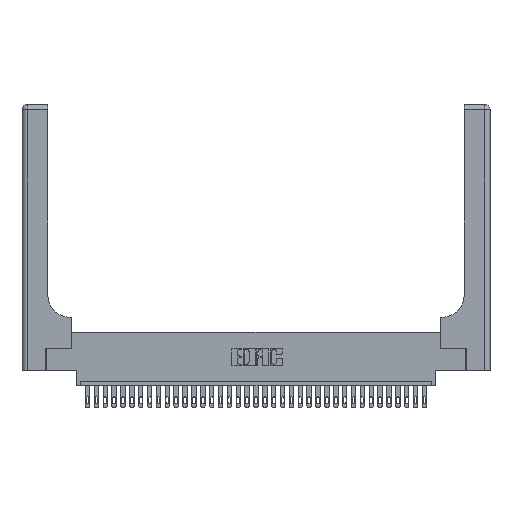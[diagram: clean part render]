
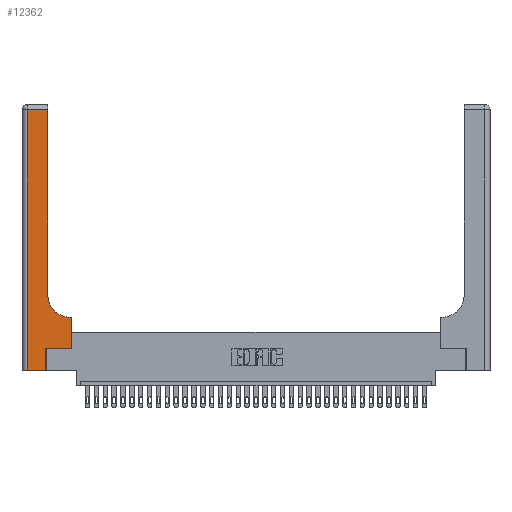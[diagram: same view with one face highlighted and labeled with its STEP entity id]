
A CAD part, top view. The second image highlights one B-rep face of the part: STEP entity #12362.
In plain terms, the highlighted planar face has unit normal (0, 0, 1).
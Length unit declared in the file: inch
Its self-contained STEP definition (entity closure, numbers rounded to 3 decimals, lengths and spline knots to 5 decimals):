
#39 = VECTOR ( 'NONE', #33072, 39.37008 ) ;
#1575 = CARTESIAN_POINT ( 'NONE',  ( 0.06, 0., 0.37 ) ) ;
#1857 = VECTOR ( 'NONE', #12751, 39.37008 ) ;
#2114 = ORIENTED_EDGE ( 'NONE', *, *, #26939, .T. ) ;
#2573 = VERTEX_POINT ( 'NONE', #28068 ) ;
#3101 = CARTESIAN_POINT ( 'NONE',  ( 0.269, 0., 0.37 ) ) ;
#4083 = VECTOR ( 'NONE', #10354, 39.37008 ) ;
#4309 = CARTESIAN_POINT ( 'NONE',  ( 0.2915, 3., 0.37 ) ) ;
#4484 = CARTESIAN_POINT ( 'NONE',  ( 0.2915, 0.85, 0.37 ) ) ;
#4776 = DIRECTION ( 'NONE',  ( 0., -1., 0. ) ) ;
#4898 = CARTESIAN_POINT ( 'NONE',  ( 0.5585, 0.25, 0.37 ) ) ;
#6067 = PLANE ( 'NONE',  #28166 ) ;
#6291 = CARTESIAN_POINT ( 'NONE',  ( 0.5415, 0.85, 0.37 ) ) ;
#6538 = DIRECTION ( 'NONE',  ( 1., 0., 0. ) ) ;
#6591 = VERTEX_POINT ( 'NONE', #14511 ) ;
#6718 = VERTEX_POINT ( 'NONE', #15034 ) ;
#6890 = FACE_OUTER_BOUND ( 'NONE', #18876, .T. ) ;
#7747 = VECTOR ( 'NONE', #26226, 39.37008 ) ;
#8608 = ORIENTED_EDGE ( 'NONE', *, *, #24534, .T. ) ;
#9350 = VERTEX_POINT ( 'NONE', #4898 ) ;
#10354 = DIRECTION ( 'NONE',  ( 1., 0., 0. ) ) ;
#10865 = CARTESIAN_POINT ( 'NONE',  ( 0.2915, 0.6, 0.37 ) ) ;
#10964 = DIRECTION ( 'NONE',  ( -1., 0., 0. ) ) ;
#11246 = EDGE_CURVE ( 'NONE', #9350, #2573, #31911, .T. ) ;
#11301 = CARTESIAN_POINT ( 'NONE',  ( 0.5585, 0.25, 0.37 ) ) ;
#12362 = ADVANCED_FACE ( 'NONE', ( #6890 ), #6067, .F. ) ;
#12525 = VECTOR ( 'NONE', #4776, 39.37008 ) ;
#12566 = ORIENTED_EDGE ( 'NONE', *, *, #16858, .T. ) ;
#12751 = DIRECTION ( 'NONE',  ( 1., 0., 0. ) ) ;
#13017 = VECTOR ( 'NONE', #10964, 39.37008 ) ;
#13457 = AXIS2_PLACEMENT_3D ( 'NONE', #6291, #27834, #6538 ) ;
#14511 = CARTESIAN_POINT ( 'NONE',  ( 0.5415, 0.6, 0.37 ) ) ;
#14887 = DIRECTION ( 'NONE',  ( 0., 1., 0. ) ) ;
#15034 = CARTESIAN_POINT ( 'NONE',  ( 0.269, 0.25, 0.37 ) ) ;
#15889 = ORIENTED_EDGE ( 'NONE', *, *, #17269, .T. ) ;
#16222 = ORIENTED_EDGE ( 'NONE', *, *, #11246, .T. ) ;
#16273 = CARTESIAN_POINT ( 'NONE',  ( 0.2915, 2.94, 0.37 ) ) ;
#16723 = CARTESIAN_POINT ( 'NONE',  ( 0.269, 0., 0.37 ) ) ;
#16858 = EDGE_CURVE ( 'NONE', #20632, #29565, #27616, .T. ) ;
#16886 = ORIENTED_EDGE ( 'NONE', *, *, #28260, .T. ) ;
#17269 = EDGE_CURVE ( 'NONE', #30854, #19351, #19565, .T. ) ;
#17406 = CIRCLE ( 'NONE', #13457, 0.25 ) ;
#17494 = ORIENTED_EDGE ( 'NONE', *, *, #26509, .T. ) ;
#17739 = LINE ( 'NONE', #16723, #39 ) ;
#18876 = EDGE_LOOP ( 'NONE', ( #15889, #2114, #27465, #12566, #16886, #17494, #16222, #8608, #31124 ) ) ;
#19351 = VERTEX_POINT ( 'NONE', #16273 ) ;
#19565 = LINE ( 'NONE', #4309, #24608 ) ;
#20366 = CARTESIAN_POINT ( 'NONE',  ( 0.269, 0.25, 0.37 ) ) ;
#20632 = VERTEX_POINT ( 'NONE', #1575 ) ;
#21831 = CARTESIAN_POINT ( 'NONE',  ( 0., 3., 0.37 ) ) ;
#21997 = EDGE_CURVE ( 'NONE', #6591, #30854, #17406, .T. ) ;
#23370 = CARTESIAN_POINT ( 'NONE',  ( 0., 2.94, 0.37 ) ) ;
#23787 = VECTOR ( 'NONE', #34190, 39.37008 ) ;
#24534 = EDGE_CURVE ( 'NONE', #2573, #6591, #28591, .T. ) ;
#24545 = LINE ( 'NONE', #23370, #7747 ) ;
#24608 = VECTOR ( 'NONE', #14887, 39.37008 ) ;
#24884 = DIRECTION ( 'NONE',  ( -1., 0., 0. ) ) ;
#25833 = CARTESIAN_POINT ( 'NONE',  ( 0.06, 3., 0.37 ) ) ;
#26226 = DIRECTION ( 'NONE',  ( -1., 0., 0. ) ) ;
#26509 = EDGE_CURVE ( 'NONE', #6718, #9350, #34383, .T. ) ;
#26939 = EDGE_CURVE ( 'NONE', #19351, #28605, #24545, .T. ) ;
#27465 = ORIENTED_EDGE ( 'NONE', *, *, #30281, .T. ) ;
#27616 = LINE ( 'NONE', #28001, #4083 ) ;
#27834 = DIRECTION ( 'NONE',  ( 0., 0., -1. ) ) ;
#28001 = CARTESIAN_POINT ( 'NONE',  ( 0., 0., 0.37 ) ) ;
#28068 = CARTESIAN_POINT ( 'NONE',  ( 0.5585, 0.6, 0.37 ) ) ;
#28166 = AXIS2_PLACEMENT_3D ( 'NONE', #21831, #30388, #24884 ) ;
#28260 = EDGE_CURVE ( 'NONE', #29565, #6718, #17739, .T. ) ;
#28591 = LINE ( 'NONE', #10865, #13017 ) ;
#28605 = VERTEX_POINT ( 'NONE', #34377 ) ;
#29565 = VERTEX_POINT ( 'NONE', #3101 ) ;
#30281 = EDGE_CURVE ( 'NONE', #28605, #20632, #33283, .T. ) ;
#30388 = DIRECTION ( 'NONE',  ( 0., 0., -1. ) ) ;
#30854 = VERTEX_POINT ( 'NONE', #4484 ) ;
#31124 = ORIENTED_EDGE ( 'NONE', *, *, #21997, .T. ) ;
#31911 = LINE ( 'NONE', #11301, #23787 ) ;
#33072 = DIRECTION ( 'NONE',  ( 0., 1., 0. ) ) ;
#33283 = LINE ( 'NONE', #25833, #12525 ) ;
#34190 = DIRECTION ( 'NONE',  ( 0., 1., 0. ) ) ;
#34377 = CARTESIAN_POINT ( 'NONE',  ( 0.06, 2.94, 0.37 ) ) ;
#34383 = LINE ( 'NONE', #20366, #1857 ) ;
